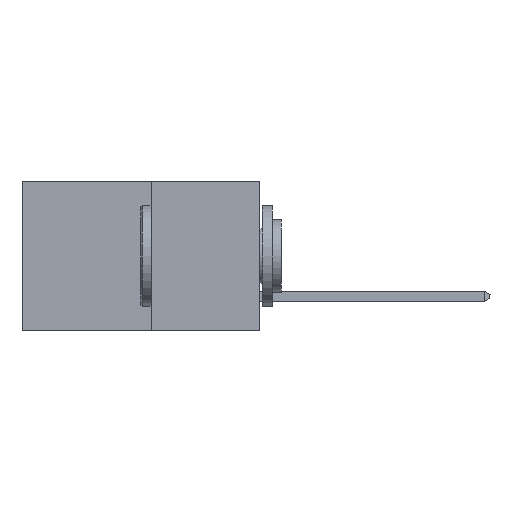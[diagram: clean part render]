
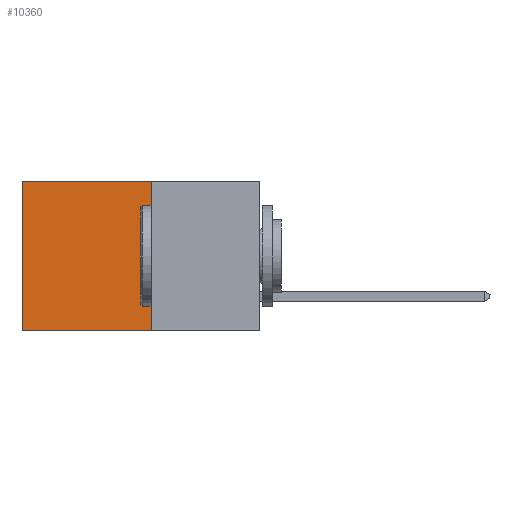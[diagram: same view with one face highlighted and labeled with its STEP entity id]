
A CAD part, left-side view. The second image highlights one B-rep face of the part: STEP entity #10360.
In plain terms, the highlighted planar face has unit normal (-1, 0, 0).
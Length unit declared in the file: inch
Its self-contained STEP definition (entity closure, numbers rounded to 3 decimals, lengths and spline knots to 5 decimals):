
#2728 = CARTESIAN_POINT ( 'NONE',  ( 0.277, 0.27, -0.37 ) ) ;
#3512 = EDGE_CURVE ( 'NONE', #17957, #21324, #7939, .T. ) ;
#3561 = DIRECTION ( 'NONE',  ( 0., 0., -1. ) ) ;
#3866 = ORIENTED_EDGE ( 'NONE', *, *, #3512, .T. ) ;
#4168 = CARTESIAN_POINT ( 'NONE',  ( 0.277, 0.27, -0.37 ) ) ;
#4805 = DIRECTION ( 'NONE',  ( 0., 0., -1. ) ) ;
#5475 = DIRECTION ( 'NONE',  ( 0., 1., 0. ) ) ;
#6019 = DIRECTION ( 'NONE',  ( 0., 0., -1. ) ) ;
#6058 = CARTESIAN_POINT ( 'NONE',  ( 0.277, 0.27, 0. ) ) ;
#6139 = AXIS2_PLACEMENT_3D ( 'NONE', #2728, #16932, #4805 ) ;
#6257 = ORIENTED_EDGE ( 'NONE', *, *, #8086, .F. ) ;
#6298 = VECTOR ( 'NONE', #3561, 39.37008 ) ;
#6662 = VECTOR ( 'NONE', #5475, 39.37008 ) ;
#7592 = CARTESIAN_POINT ( 'NONE',  ( 0.277, 0.27, -0.37 ) ) ;
#7939 = LINE ( 'NONE', #6058, #6662 ) ;
#8086 = EDGE_CURVE ( 'NONE', #17957, #15125, #23032, .T. ) ;
#9564 = VECTOR ( 'NONE', #9638, 39.37008 ) ;
#9638 = DIRECTION ( 'NONE',  ( 0., 1., 0. ) ) ;
#10360 = ADVANCED_FACE ( 'NONE', ( #15623 ), #14901, .F. ) ;
#12178 = CARTESIAN_POINT ( 'NONE',  ( 0.277, 0.59, -0.37 ) ) ;
#14901 = PLANE ( 'NONE',  #6139 ) ;
#15125 = VERTEX_POINT ( 'NONE', #4168 ) ;
#15576 = EDGE_LOOP ( 'NONE', ( #21200, #19088, #6257, #3866 ) ) ;
#15623 = FACE_OUTER_BOUND ( 'NONE', #15576, .T. ) ;
#16271 = CARTESIAN_POINT ( 'NONE',  ( 0.277, 0.27, 0. ) ) ;
#16932 = DIRECTION ( 'NONE',  ( 1., 0., 0. ) ) ;
#17957 = VERTEX_POINT ( 'NONE', #16271 ) ;
#18080 = CARTESIAN_POINT ( 'NONE',  ( 0.277, 0.59, -0.37 ) ) ;
#19088 = ORIENTED_EDGE ( 'NONE', *, *, #20962, .F. ) ;
#20962 = EDGE_CURVE ( 'NONE', #15125, #21128, #23338, .T. ) ;
#21128 = VERTEX_POINT ( 'NONE', #12178 ) ;
#21200 = ORIENTED_EDGE ( 'NONE', *, *, #22481, .T. ) ;
#21324 = VERTEX_POINT ( 'NONE', #22661 ) ;
#22481 = EDGE_CURVE ( 'NONE', #21324, #21128, #25208, .T. ) ;
#22661 = CARTESIAN_POINT ( 'NONE',  ( 0.277, 0.59, 0. ) ) ;
#23032 = LINE ( 'NONE', #7592, #6298 ) ;
#23338 = LINE ( 'NONE', #25723, #9564 ) ;
#24587 = VECTOR ( 'NONE', #6019, 39.37008 ) ;
#25208 = LINE ( 'NONE', #18080, #24587 ) ;
#25723 = CARTESIAN_POINT ( 'NONE',  ( 0.277, 0.27, -0.37 ) ) ;
